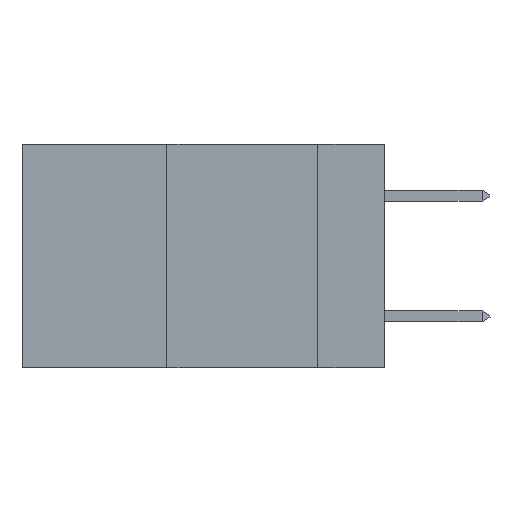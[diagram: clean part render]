
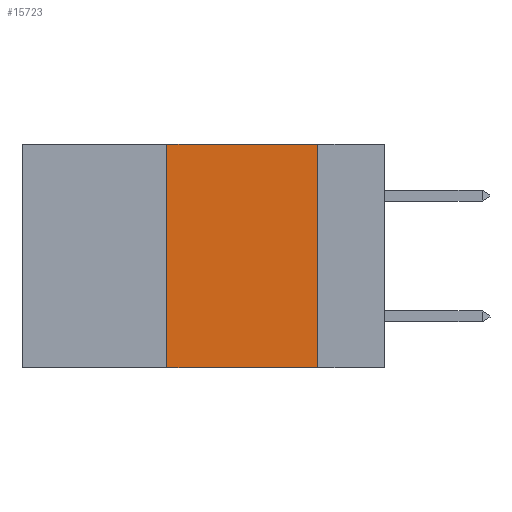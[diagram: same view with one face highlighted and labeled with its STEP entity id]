
A CAD part, left-side view. The second image highlights one B-rep face of the part: STEP entity #15723.
In plain terms, the highlighted planar face has unit normal (-1, 0, 0).
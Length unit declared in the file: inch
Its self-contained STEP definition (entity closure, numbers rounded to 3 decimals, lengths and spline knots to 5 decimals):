
#1864 = EDGE_CURVE ( 'NONE', #19430, #16370, #9800, .T. ) ;
#2370 = VERTEX_POINT ( 'NONE', #23427 ) ;
#4555 = DIRECTION ( 'NONE',  ( 0., -1., 0. ) ) ;
#6241 = VECTOR ( 'NONE', #14519, 39.37008 ) ;
#6801 = CARTESIAN_POINT ( 'NONE',  ( 0., 0.11, 0. ) ) ;
#8512 = EDGE_LOOP ( 'NONE', ( #11773, #22126, #12969, #13559 ) ) ;
#9800 = LINE ( 'NONE', #22103, #23902 ) ;
#10113 = VECTOR ( 'NONE', #15712, 39.37008 ) ;
#10588 = CARTESIAN_POINT ( 'NONE',  ( 0., 0.6, 0. ) ) ;
#11773 = ORIENTED_EDGE ( 'NONE', *, *, #19378, .F. ) ;
#11921 = CARTESIAN_POINT ( 'NONE',  ( 0., 0.36, 0. ) ) ;
#12464 = DIRECTION ( 'NONE',  ( 0., 0., -1. ) ) ;
#12969 = ORIENTED_EDGE ( 'NONE', *, *, #18145, .F. ) ;
#13559 = ORIENTED_EDGE ( 'NONE', *, *, #21735, .T. ) ;
#14519 = DIRECTION ( 'NONE',  ( 0., 0., -1. ) ) ;
#14705 = CARTESIAN_POINT ( 'NONE',  ( 0., 0.36, -0.37 ) ) ;
#15095 = LINE ( 'NONE', #11921, #10113 ) ;
#15712 = DIRECTION ( 'NONE',  ( 0., 0., 1. ) ) ;
#15723 = ADVANCED_FACE ( 'NONE', ( #17204 ), #21609, .F. ) ;
#15853 = VERTEX_POINT ( 'NONE', #14705 ) ;
#16013 = CARTESIAN_POINT ( 'NONE',  ( 0., 0.6, -0.37 ) ) ;
#16344 = LINE ( 'NONE', #23557, #6241 ) ;
#16370 = VERTEX_POINT ( 'NONE', #6801 ) ;
#16443 = CARTESIAN_POINT ( 'NONE',  ( 0., 0.36, 0. ) ) ;
#17204 = FACE_OUTER_BOUND ( 'NONE', #8512, .T. ) ;
#18145 = EDGE_CURVE ( 'NONE', #15853, #19430, #15095, .T. ) ;
#18602 = VECTOR ( 'NONE', #4555, 39.37008 ) ;
#19378 = EDGE_CURVE ( 'NONE', #16370, #2370, #16344, .T. ) ;
#19430 = VERTEX_POINT ( 'NONE', #16443 ) ;
#20874 = AXIS2_PLACEMENT_3D ( 'NONE', #10588, #23422, #12464 ) ;
#21609 = PLANE ( 'NONE',  #20874 ) ;
#21735 = EDGE_CURVE ( 'NONE', #15853, #2370, #22773, .T. ) ;
#22103 = CARTESIAN_POINT ( 'NONE',  ( 0., 0.6, 0. ) ) ;
#22126 = ORIENTED_EDGE ( 'NONE', *, *, #1864, .F. ) ;
#22773 = LINE ( 'NONE', #16013, #18602 ) ;
#23422 = DIRECTION ( 'NONE',  ( 1., 0., 0. ) ) ;
#23427 = CARTESIAN_POINT ( 'NONE',  ( 0., 0.11, -0.37 ) ) ;
#23557 = CARTESIAN_POINT ( 'NONE',  ( 0., 0.11, 0. ) ) ;
#23902 = VECTOR ( 'NONE', #23945, 39.37008 ) ;
#23945 = DIRECTION ( 'NONE',  ( 0., -1., 0. ) ) ;
